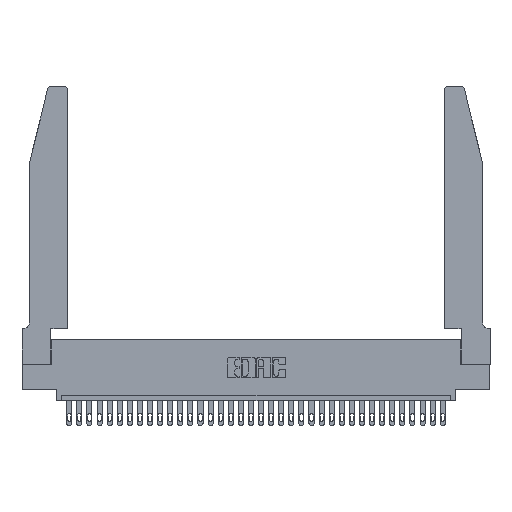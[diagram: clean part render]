
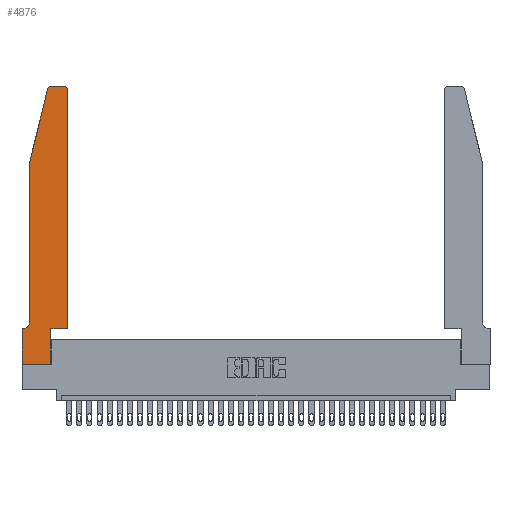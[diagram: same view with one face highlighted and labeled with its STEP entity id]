
A CAD part, top view. The second image highlights one B-rep face of the part: STEP entity #4876.
In plain terms, the highlighted planar face has unit normal (0, 0, 1).
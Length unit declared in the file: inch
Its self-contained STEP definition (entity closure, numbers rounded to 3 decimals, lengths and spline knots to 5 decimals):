
#247 = DIRECTION ( 'NONE',  ( -1., 0., 0. ) ) ;
#430 = EDGE_CURVE ( 'NONE', #28580, #28764, #4724, .T. ) ;
#579 = CARTESIAN_POINT ( 'NONE',  ( 0., 0., 0.37 ) ) ;
#663 = EDGE_CURVE ( 'NONE', #16146, #14012, #5516, .T. ) ;
#1327 = DIRECTION ( 'NONE',  ( 1., 0., 0. ) ) ;
#1596 = DIRECTION ( 'NONE',  ( 0., -1., 0. ) ) ;
#1652 = EDGE_CURVE ( 'NONE', #31918, #28580, #29643, .T. ) ;
#1920 = AXIS2_PLACEMENT_3D ( 'NONE', #9554, #4579, #6782 ) ;
#1958 = CARTESIAN_POINT ( 'NONE',  ( 0.4205, 2.75, 0.37 ) ) ;
#2038 = DIRECTION ( 'NONE',  ( 0., 0., -1. ) ) ;
#2679 = ORIENTED_EDGE ( 'NONE', *, *, #23593, .T. ) ;
#3240 = DIRECTION ( 'NONE',  ( 0., -1., 0. ) ) ;
#3508 = AXIS2_PLACEMENT_3D ( 'NONE', #18963, #29631, #8565 ) ;
#3545 = CARTESIAN_POINT ( 'NONE',  ( 0.0755, 2., 0.37 ) ) ;
#3572 = ORIENTED_EDGE ( 'NONE', *, *, #430, .T. ) ;
#3594 = EDGE_CURVE ( 'NONE', #31449, #16850, #5369, .T. ) ;
#3637 = VERTEX_POINT ( 'NONE', #3925 ) ;
#3715 = EDGE_LOOP ( 'NONE', ( #11988, #13213, #6247, #13027, #12416, #23164, #3572, #2679, #30068, #19563, #22782, #25968 ) ) ;
#3925 = CARTESIAN_POINT ( 'NONE',  ( 0.4505, 0.35, 0.37 ) ) ;
#4149 = DIRECTION ( 'NONE',  ( 1., 0., 0. ) ) ;
#4579 = DIRECTION ( 'NONE',  ( 0., 0., 1. ) ) ;
#4686 = VECTOR ( 'NONE', #32983, 39.37008 ) ;
#4724 = LINE ( 'NONE', #579, #17023 ) ;
#4876 = ADVANCED_FACE ( 'NONE', ( #11035 ), #24235, .T. ) ;
#4906 = CARTESIAN_POINT ( 'NONE',  ( 0., 0.35, 0.37 ) ) ;
#5091 = CARTESIAN_POINT ( 'NONE',  ( 0.284, 2.75, 0.37 ) ) ;
#5327 = VERTEX_POINT ( 'NONE', #25593 ) ;
#5369 = CIRCLE ( 'NONE', #20609, 0.03 ) ;
#5516 = CIRCLE ( 'NONE', #1920, 0.03 ) ;
#6247 = ORIENTED_EDGE ( 'NONE', *, *, #32896, .T. ) ;
#6443 = CARTESIAN_POINT ( 'NONE',  ( 0.0755, 2., 0.37 ) ) ;
#6447 = EDGE_CURVE ( 'NONE', #5327, #17055, #26120, .T. ) ;
#6782 = DIRECTION ( 'NONE',  ( 1., 0., 0. ) ) ;
#7174 = LINE ( 'NONE', #27840, #4686 ) ;
#7284 = CARTESIAN_POINT ( 'NONE',  ( 0.0055, 0.42, 0.37 ) ) ;
#7395 = CARTESIAN_POINT ( 'NONE',  ( 0.25487, 2.72718, 0.37 ) ) ;
#8148 = VECTOR ( 'NONE', #1327, 39.37008 ) ;
#8565 = DIRECTION ( 'NONE',  ( 1., 0., 0. ) ) ;
#8950 = VECTOR ( 'NONE', #16505, 39.37008 ) ;
#9554 = CARTESIAN_POINT ( 'NONE',  ( 0.4205, 2.72, 0.37 ) ) ;
#10887 = DIRECTION ( 'NONE',  ( 0., 1., 0. ) ) ;
#11035 = FACE_OUTER_BOUND ( 'NONE', #3715, .T. ) ;
#11168 = CARTESIAN_POINT ( 'NONE',  ( 0.0755, 0.42, 0.37 ) ) ;
#11709 = CARTESIAN_POINT ( 'NONE',  ( 0.2865, 0.35, 0.37 ) ) ;
#11802 = LINE ( 'NONE', #21284, #33527 ) ;
#11988 = ORIENTED_EDGE ( 'NONE', *, *, #32068, .T. ) ;
#12416 = ORIENTED_EDGE ( 'NONE', *, *, #27128, .T. ) ;
#13027 = ORIENTED_EDGE ( 'NONE', *, *, #20024, .T. ) ;
#13146 = CARTESIAN_POINT ( 'NONE',  ( 0.4505, 2.72, 0.37 ) ) ;
#13213 = ORIENTED_EDGE ( 'NONE', *, *, #3594, .T. ) ;
#13597 = AXIS2_PLACEMENT_3D ( 'NONE', #7284, #2038, #25632 ) ;
#14012 = VERTEX_POINT ( 'NONE', #1958 ) ;
#14134 = VECTOR ( 'NONE', #247, 39.37008 ) ;
#14536 = DIRECTION ( 'NONE',  ( 0., 0., 1. ) ) ;
#14882 = VERTEX_POINT ( 'NONE', #6443 ) ;
#16146 = VERTEX_POINT ( 'NONE', #13146 ) ;
#16365 = CARTESIAN_POINT ( 'NONE',  ( 0., 0., 0.37 ) ) ;
#16505 = DIRECTION ( 'NONE',  ( 1., 0., 0. ) ) ;
#16738 = LINE ( 'NONE', #18979, #8950 ) ;
#16850 = VERTEX_POINT ( 'NONE', #7395 ) ;
#17023 = VECTOR ( 'NONE', #3240, 39.37008 ) ;
#17055 = VERTEX_POINT ( 'NONE', #11709 ) ;
#17626 = VECTOR ( 'NONE', #23977, 39.37008 ) ;
#18042 = DIRECTION ( 'NONE',  ( 0., 1., 0. ) ) ;
#18963 = CARTESIAN_POINT ( 'NONE',  ( 0., 0.35, 0.37 ) ) ;
#18979 = CARTESIAN_POINT ( 'NONE',  ( 0.4505, 0.35, 0.37 ) ) ;
#19360 = CARTESIAN_POINT ( 'NONE',  ( 0.0055, 0.35, 0.37 ) ) ;
#19563 = ORIENTED_EDGE ( 'NONE', *, *, #26316, .T. ) ;
#20024 = EDGE_CURVE ( 'NONE', #14882, #23629, #30431, .T. ) ;
#20068 = LINE ( 'NONE', #26507, #17626 ) ;
#20365 = VECTOR ( 'NONE', #18042, 39.37008 ) ;
#20609 = AXIS2_PLACEMENT_3D ( 'NONE', #30142, #14536, #4149 ) ;
#21284 = CARTESIAN_POINT ( 'NONE',  ( 0.4505, 0.35, 0.37 ) ) ;
#21584 = CARTESIAN_POINT ( 'NONE',  ( 0.0755, 0.35, 0.37 ) ) ;
#22402 = CIRCLE ( 'NONE', #13597, 0.07 ) ;
#22782 = ORIENTED_EDGE ( 'NONE', *, *, #26278, .T. ) ;
#22930 = CARTESIAN_POINT ( 'NONE',  ( 0.2865, 0.35, 0.37 ) ) ;
#23164 = ORIENTED_EDGE ( 'NONE', *, *, #1652, .T. ) ;
#23593 = EDGE_CURVE ( 'NONE', #28764, #5327, #27814, .T. ) ;
#23629 = VERTEX_POINT ( 'NONE', #11168 ) ;
#23977 = DIRECTION ( 'NONE',  ( -0.239, -0.971, 0. ) ) ;
#24235 = PLANE ( 'NONE',  #3508 ) ;
#25593 = CARTESIAN_POINT ( 'NONE',  ( 0.2865, 0., 0.37 ) ) ;
#25632 = DIRECTION ( 'NONE',  ( -1., 0., 0. ) ) ;
#25968 = ORIENTED_EDGE ( 'NONE', *, *, #663, .T. ) ;
#26120 = LINE ( 'NONE', #22930, #20365 ) ;
#26278 = EDGE_CURVE ( 'NONE', #3637, #16146, #11802, .T. ) ;
#26316 = EDGE_CURVE ( 'NONE', #17055, #3637, #16738, .T. ) ;
#26507 = CARTESIAN_POINT ( 'NONE',  ( 0.0755, 2., 0.37 ) ) ;
#27128 = EDGE_CURVE ( 'NONE', #23629, #31918, #22402, .T. ) ;
#27814 = LINE ( 'NONE', #32919, #8148 ) ;
#27840 = CARTESIAN_POINT ( 'NONE',  ( 0.2605, 2.75, 0.37 ) ) ;
#28580 = VERTEX_POINT ( 'NONE', #4906 ) ;
#28764 = VERTEX_POINT ( 'NONE', #16365 ) ;
#29237 = VECTOR ( 'NONE', #1596, 39.37008 ) ;
#29631 = DIRECTION ( 'NONE',  ( 0., 0., 1. ) ) ;
#29643 = LINE ( 'NONE', #21584, #14134 ) ;
#30068 = ORIENTED_EDGE ( 'NONE', *, *, #6447, .T. ) ;
#30142 = CARTESIAN_POINT ( 'NONE',  ( 0.284, 2.72, 0.37 ) ) ;
#30431 = LINE ( 'NONE', #3545, #29237 ) ;
#31449 = VERTEX_POINT ( 'NONE', #5091 ) ;
#31918 = VERTEX_POINT ( 'NONE', #19360 ) ;
#32068 = EDGE_CURVE ( 'NONE', #14012, #31449, #7174, .T. ) ;
#32896 = EDGE_CURVE ( 'NONE', #16850, #14882, #20068, .T. ) ;
#32919 = CARTESIAN_POINT ( 'NONE',  ( 0., 0., 0.37 ) ) ;
#32983 = DIRECTION ( 'NONE',  ( -1., 0., 0. ) ) ;
#33527 = VECTOR ( 'NONE', #10887, 39.37008 ) ;
